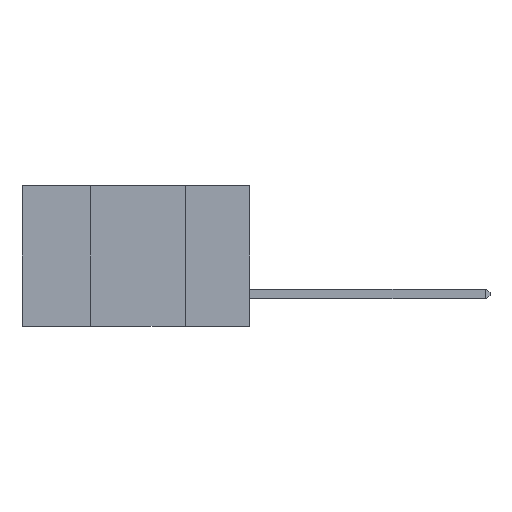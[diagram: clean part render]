
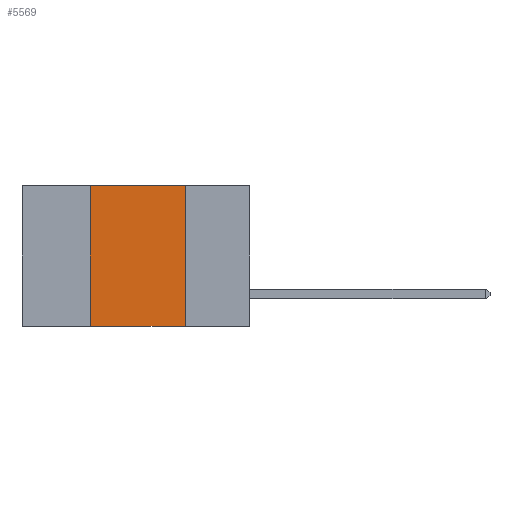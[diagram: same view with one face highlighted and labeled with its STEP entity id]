
A CAD part, left-side view. The second image highlights one B-rep face of the part: STEP entity #5569.
In plain terms, the highlighted planar face has unit normal (-1, 0, 0).
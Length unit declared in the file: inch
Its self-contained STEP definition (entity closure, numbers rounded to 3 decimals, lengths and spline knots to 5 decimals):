
#270 = VERTEX_POINT ( 'NONE', #10725 ) ;
#492 = CARTESIAN_POINT ( 'NONE',  ( 0., 0.6, -0.37 ) ) ;
#592 = DIRECTION ( 'NONE',  ( 0., -1., 0. ) ) ;
#642 = PLANE ( 'NONE',  #3098 ) ;
#1154 = VERTEX_POINT ( 'NONE', #3655 ) ;
#1190 = CARTESIAN_POINT ( 'NONE',  ( 0., 0.6, 0. ) ) ;
#1679 = CARTESIAN_POINT ( 'NONE',  ( 0., 0.6, 0. ) ) ;
#2496 = VECTOR ( 'NONE', #5266, 39.37008 ) ;
#2693 = DIRECTION ( 'NONE',  ( 1., 0., 0. ) ) ;
#2926 = VERTEX_POINT ( 'NONE', #10659 ) ;
#2963 = VERTEX_POINT ( 'NONE', #8732 ) ;
#3057 = DIRECTION ( 'NONE',  ( 0., 0., 1. ) ) ;
#3098 = AXIS2_PLACEMENT_3D ( 'NONE', #1679, #2693, #9573 ) ;
#3331 = LINE ( 'NONE', #12572, #3958 ) ;
#3369 = DIRECTION ( 'NONE',  ( 0., 0., -1. ) ) ;
#3501 = LINE ( 'NONE', #492, #10927 ) ;
#3655 = CARTESIAN_POINT ( 'NONE',  ( 0., 0.42, 0. ) ) ;
#3958 = VECTOR ( 'NONE', #3057, 39.37008 ) ;
#4369 = LINE ( 'NONE', #10184, #11709 ) ;
#4488 = EDGE_CURVE ( 'NONE', #2926, #2963, #3501, .T. ) ;
#5189 = LINE ( 'NONE', #1190, #2496 ) ;
#5203 = EDGE_CURVE ( 'NONE', #2926, #1154, #3331, .T. ) ;
#5266 = DIRECTION ( 'NONE',  ( 0., -1., 0. ) ) ;
#5569 = ADVANCED_FACE ( 'NONE', ( #8308 ), #642, .F. ) ;
#6546 = EDGE_CURVE ( 'NONE', #270, #2963, #4369, .T. ) ;
#6989 = ORIENTED_EDGE ( 'NONE', *, *, #4488, .T. ) ;
#7102 = EDGE_CURVE ( 'NONE', #1154, #270, #5189, .T. ) ;
#8308 = FACE_OUTER_BOUND ( 'NONE', #10354, .T. ) ;
#8732 = CARTESIAN_POINT ( 'NONE',  ( 0., 0.17, -0.37 ) ) ;
#9573 = DIRECTION ( 'NONE',  ( 0., 0., -1. ) ) ;
#10184 = CARTESIAN_POINT ( 'NONE',  ( 0., 0.17, 0. ) ) ;
#10354 = EDGE_LOOP ( 'NONE', ( #10528, #10808, #11931, #6989 ) ) ;
#10528 = ORIENTED_EDGE ( 'NONE', *, *, #6546, .F. ) ;
#10659 = CARTESIAN_POINT ( 'NONE',  ( 0., 0.42, -0.37 ) ) ;
#10725 = CARTESIAN_POINT ( 'NONE',  ( 0., 0.17, 0. ) ) ;
#10808 = ORIENTED_EDGE ( 'NONE', *, *, #7102, .F. ) ;
#10927 = VECTOR ( 'NONE', #592, 39.37008 ) ;
#11709 = VECTOR ( 'NONE', #3369, 39.37008 ) ;
#11931 = ORIENTED_EDGE ( 'NONE', *, *, #5203, .F. ) ;
#12572 = CARTESIAN_POINT ( 'NONE',  ( 0., 0.42, 0. ) ) ;
